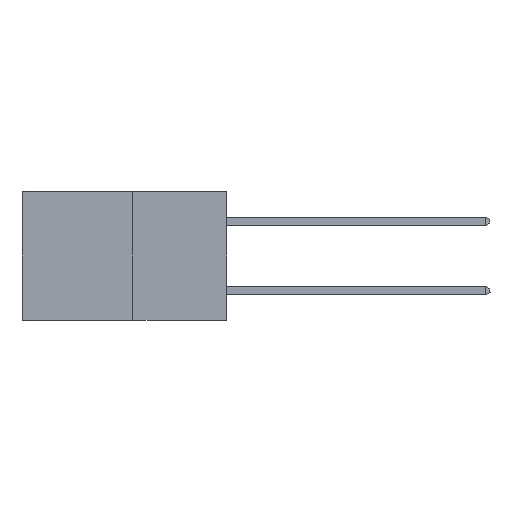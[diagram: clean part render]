
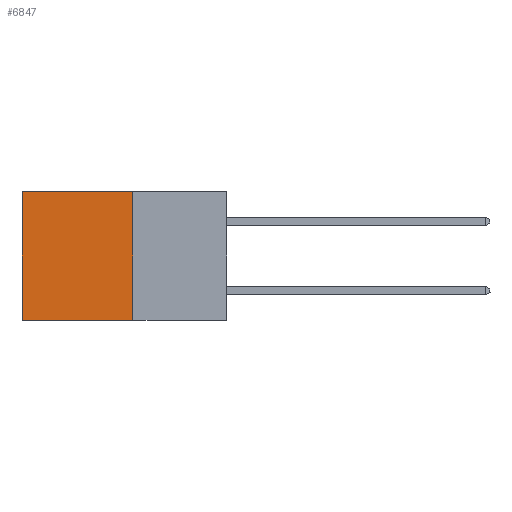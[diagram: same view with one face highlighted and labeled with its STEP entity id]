
A CAD part, left-side view. The second image highlights one B-rep face of the part: STEP entity #6847.
In plain terms, the highlighted planar face has unit normal (-1, 0, 0).
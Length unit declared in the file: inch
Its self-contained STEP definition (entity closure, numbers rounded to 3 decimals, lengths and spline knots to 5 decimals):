
#209 = VECTOR ( 'NONE', #2701, 39.37008 ) ;
#351 = VERTEX_POINT ( 'NONE', #8836 ) ;
#491 = DIRECTION ( 'NONE',  ( 0., 1., 0. ) ) ;
#650 = DIRECTION ( 'NONE',  ( 0., 0., -1. ) ) ;
#945 = ORIENTED_EDGE ( 'NONE', *, *, #13888, .F. ) ;
#1454 = CARTESIAN_POINT ( 'NONE',  ( 0.277, 0.27, -0.37 ) ) ;
#1791 = EDGE_CURVE ( 'NONE', #10459, #351, #10600, .T. ) ;
#2515 = VERTEX_POINT ( 'NONE', #16661 ) ;
#2701 = DIRECTION ( 'NONE',  ( 0., 1., 0. ) ) ;
#3355 = CARTESIAN_POINT ( 'NONE',  ( 0.277, 0.27, -0.37 ) ) ;
#3410 = LINE ( 'NONE', #1454, #13408 ) ;
#3436 = AXIS2_PLACEMENT_3D ( 'NONE', #9310, #9261, #9226 ) ;
#4887 = CARTESIAN_POINT ( 'NONE',  ( 0.277, 0.27, -0.37 ) ) ;
#5144 = VERTEX_POINT ( 'NONE', #5298 ) ;
#5298 = CARTESIAN_POINT ( 'NONE',  ( 0.277, 0.59, 0. ) ) ;
#6418 = ORIENTED_EDGE ( 'NONE', *, *, #10609, .T. ) ;
#6568 = VECTOR ( 'NONE', #650, 39.37008 ) ;
#6847 = ADVANCED_FACE ( 'NONE', ( #15900 ), #9608, .F. ) ;
#7751 = ORIENTED_EDGE ( 'NONE', *, *, #12674, .T. ) ;
#8836 = CARTESIAN_POINT ( 'NONE',  ( 0.277, 0.59, -0.37 ) ) ;
#9226 = DIRECTION ( 'NONE',  ( 0., 0., -1. ) ) ;
#9255 = DIRECTION ( 'NONE',  ( 0., 0., -1. ) ) ;
#9261 = DIRECTION ( 'NONE',  ( 1., 0., 0. ) ) ;
#9310 = CARTESIAN_POINT ( 'NONE',  ( 0.277, 0.27, -0.37 ) ) ;
#9608 = PLANE ( 'NONE',  #3436 ) ;
#9619 = CARTESIAN_POINT ( 'NONE',  ( 0.277, 0.27, 0. ) ) ;
#10459 = VERTEX_POINT ( 'NONE', #3355 ) ;
#10600 = LINE ( 'NONE', #4887, #209 ) ;
#10609 = EDGE_CURVE ( 'NONE', #2515, #5144, #15215, .T. ) ;
#12674 = EDGE_CURVE ( 'NONE', #5144, #351, #13505, .T. ) ;
#13408 = VECTOR ( 'NONE', #9255, 39.37008 ) ;
#13505 = LINE ( 'NONE', #16189, #6568 ) ;
#13888 = EDGE_CURVE ( 'NONE', #2515, #10459, #3410, .T. ) ;
#14521 = EDGE_LOOP ( 'NONE', ( #7751, #16697, #945, #6418 ) ) ;
#14825 = VECTOR ( 'NONE', #491, 39.37008 ) ;
#15215 = LINE ( 'NONE', #9619, #14825 ) ;
#15900 = FACE_OUTER_BOUND ( 'NONE', #14521, .T. ) ;
#16189 = CARTESIAN_POINT ( 'NONE',  ( 0.277, 0.59, -0.37 ) ) ;
#16661 = CARTESIAN_POINT ( 'NONE',  ( 0.277, 0.27, 0. ) ) ;
#16697 = ORIENTED_EDGE ( 'NONE', *, *, #1791, .F. ) ;
